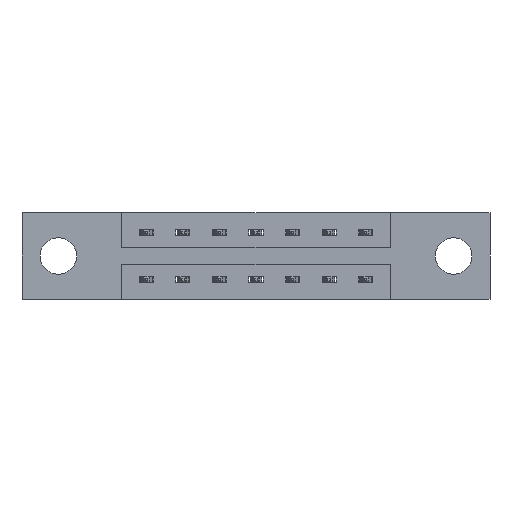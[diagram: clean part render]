
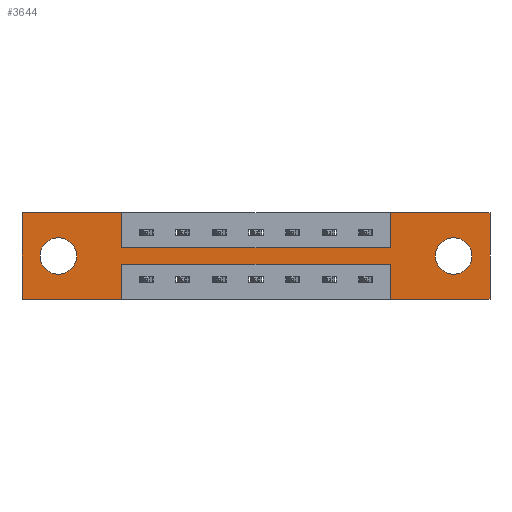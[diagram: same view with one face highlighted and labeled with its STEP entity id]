
A CAD part, front view. The second image highlights one B-rep face of the part: STEP entity #3644.
In plain terms, the highlighted planar face has unit normal (0, -1, 0).
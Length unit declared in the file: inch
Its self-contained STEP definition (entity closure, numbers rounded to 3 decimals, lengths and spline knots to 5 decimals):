
#55 = EDGE_CURVE ( 'NONE', #8489, #938, #3710, .T. ) ;
#57 = CIRCLE ( 'NONE', #2576, 0.078 ) ;
#244 = EDGE_CURVE ( 'NONE', #3128, #1356, #6852, .T. ) ;
#360 = DIRECTION ( 'NONE',  ( 0., 1., 0. ) ) ;
#415 = DIRECTION ( 'NONE',  ( 1., 0., 0. ) ) ;
#687 = CARTESIAN_POINT ( 'NONE',  ( 0.155, 0., -0.185 ) ) ;
#725 = ORIENTED_EDGE ( 'NONE', *, *, #8463, .F. ) ;
#742 = ORIENTED_EDGE ( 'NONE', *, *, #244, .F. ) ;
#936 = LINE ( 'NONE', #1928, #2148 ) ;
#938 = VERTEX_POINT ( 'NONE', #7588 ) ;
#1130 = VERTEX_POINT ( 'NONE', #7873 ) ;
#1139 = ORIENTED_EDGE ( 'NONE', *, *, #9358, .F. ) ;
#1258 = DIRECTION ( 'NONE',  ( 0., 0., -1. ) ) ;
#1273 = VERTEX_POINT ( 'NONE', #8137 ) ;
#1356 = VERTEX_POINT ( 'NONE', #8994 ) ;
#1363 = EDGE_CURVE ( 'NONE', #7851, #3679, #5012, .T. ) ;
#1532 = LINE ( 'NONE', #3522, #5230 ) ;
#1639 = DIRECTION ( 'NONE',  ( 0., 0., 1. ) ) ;
#1818 = EDGE_CURVE ( 'NONE', #1130, #3128, #1532, .T. ) ;
#1835 = CARTESIAN_POINT ( 'NONE',  ( 0.425, 0., -0.15 ) ) ;
#1843 = LINE ( 'NONE', #5251, #6759 ) ;
#1888 = CIRCLE ( 'NONE', #5124, 0.078 ) ;
#1928 = CARTESIAN_POINT ( 'NONE',  ( 1.573, 0., 0. ) ) ;
#2063 = LINE ( 'NONE', #8984, #8922 ) ;
#2148 = VECTOR ( 'NONE', #2625, 39.37008 ) ;
#2162 = CARTESIAN_POINT ( 'NONE',  ( 0., 0., -0.37 ) ) ;
#2202 = AXIS2_PLACEMENT_3D ( 'NONE', #687, #4536, #9292 ) ;
#2242 = DIRECTION ( 'NONE',  ( 0., 0., -1. ) ) ;
#2257 = FACE_BOUND ( 'NONE', #9758, .T. ) ;
#2281 = VERTEX_POINT ( 'NONE', #3507 ) ;
#2293 = VECTOR ( 'NONE', #8627, 39.37008 ) ;
#2341 = LINE ( 'NONE', #7814, #8841 ) ;
#2391 = VECTOR ( 'NONE', #5504, 39.37008 ) ;
#2440 = CARTESIAN_POINT ( 'NONE',  ( 1.573, 0., -0.37 ) ) ;
#2482 = VECTOR ( 'NONE', #4920, 39.37008 ) ;
#2576 = AXIS2_PLACEMENT_3D ( 'NONE', #2961, #6100, #4582 ) ;
#2597 = CARTESIAN_POINT ( 'NONE',  ( 0., 0., -0.37 ) ) ;
#2625 = DIRECTION ( 'NONE',  ( 0., 0., 1. ) ) ;
#2782 = VECTOR ( 'NONE', #5097, 39.37008 ) ;
#2894 = VERTEX_POINT ( 'NONE', #5723 ) ;
#2911 = EDGE_LOOP ( 'NONE', ( #9784, #5917 ) ) ;
#2961 = CARTESIAN_POINT ( 'NONE',  ( 0.155, 0., -0.185 ) ) ;
#2973 = ORIENTED_EDGE ( 'NONE', *, *, #6583, .F. ) ;
#3128 = VERTEX_POINT ( 'NONE', #8441 ) ;
#3323 = VECTOR ( 'NONE', #7646, 39.37008 ) ;
#3328 = AXIS2_PLACEMENT_3D ( 'NONE', #8236, #6020, #5959 ) ;
#3358 = VECTOR ( 'NONE', #8349, 39.37008 ) ;
#3507 = CARTESIAN_POINT ( 'NONE',  ( 1.573, 0., -0.15 ) ) ;
#3522 = CARTESIAN_POINT ( 'NONE',  ( 1.998, 0., 0. ) ) ;
#3532 = EDGE_CURVE ( 'NONE', #7318, #4775, #57, .T. ) ;
#3644 = ADVANCED_FACE ( 'NONE', ( #9954, #2257, #4858 ), #6828, .T. ) ;
#3679 = VERTEX_POINT ( 'NONE', #5228 ) ;
#3710 = LINE ( 'NONE', #8182, #2782 ) ;
#3792 = LINE ( 'NONE', #4571, #3323 ) ;
#4069 = ORIENTED_EDGE ( 'NONE', *, *, #9150, .F. ) ;
#4127 = CARTESIAN_POINT ( 'NONE',  ( 0., 0., 0. ) ) ;
#4367 = EDGE_CURVE ( 'NONE', #3679, #7851, #1888, .T. ) ;
#4536 = DIRECTION ( 'NONE',  ( 0., 1., 0. ) ) ;
#4571 = CARTESIAN_POINT ( 'NONE',  ( 0., 0., -0.37 ) ) ;
#4582 = DIRECTION ( 'NONE',  ( 0., 0., 1. ) ) ;
#4628 = EDGE_CURVE ( 'NONE', #4775, #7318, #9238, .T. ) ;
#4639 = ORIENTED_EDGE ( 'NONE', *, *, #1818, .F. ) ;
#4667 = CARTESIAN_POINT ( 'NONE',  ( 0., 0., 0. ) ) ;
#4775 = VERTEX_POINT ( 'NONE', #7078 ) ;
#4822 = CARTESIAN_POINT ( 'NONE',  ( 1.843, 0., -0.185 ) ) ;
#4858 = FACE_OUTER_BOUND ( 'NONE', #6739, .T. ) ;
#4920 = DIRECTION ( 'NONE',  ( 0., 0., 1. ) ) ;
#5012 = CIRCLE ( 'NONE', #3328, 0.078 ) ;
#5097 = DIRECTION ( 'NONE',  ( 1., 0., 0. ) ) ;
#5124 = AXIS2_PLACEMENT_3D ( 'NONE', #4822, #360, #7941 ) ;
#5191 = VERTEX_POINT ( 'NONE', #9258 ) ;
#5228 = CARTESIAN_POINT ( 'NONE',  ( 1.843, 0., -0.107 ) ) ;
#5230 = VECTOR ( 'NONE', #1258, 39.37008 ) ;
#5251 = CARTESIAN_POINT ( 'NONE',  ( 0., 0., 0. ) ) ;
#5385 = ORIENTED_EDGE ( 'NONE', *, *, #55, .F. ) ;
#5395 = EDGE_CURVE ( 'NONE', #6432, #8489, #7751, .T. ) ;
#5457 = ORIENTED_EDGE ( 'NONE', *, *, #4628, .T. ) ;
#5504 = DIRECTION ( 'NONE',  ( 0., 0., -1. ) ) ;
#5588 = CARTESIAN_POINT ( 'NONE',  ( 1.843, 0., -0.263 ) ) ;
#5723 = CARTESIAN_POINT ( 'NONE',  ( 0.425, 0., -0.22 ) ) ;
#5917 = ORIENTED_EDGE ( 'NONE', *, *, #1363, .T. ) ;
#5959 = DIRECTION ( 'NONE',  ( 0., 0., -1. ) ) ;
#6020 = DIRECTION ( 'NONE',  ( 0., 1., 0. ) ) ;
#6024 = ORIENTED_EDGE ( 'NONE', *, *, #9821, .F. ) ;
#6059 = EDGE_CURVE ( 'NONE', #938, #8451, #2341, .T. ) ;
#6100 = DIRECTION ( 'NONE',  ( 0., 1., 0. ) ) ;
#6432 = VERTEX_POINT ( 'NONE', #2597 ) ;
#6583 = EDGE_CURVE ( 'NONE', #9406, #1130, #1843, .T. ) ;
#6615 = LINE ( 'NONE', #7100, #2293 ) ;
#6739 = EDGE_LOOP ( 'NONE', ( #9679, #725, #6024, #742, #4639, #2973, #4069, #7630, #7072, #5385, #9112, #1139 ) ) ;
#6759 = VECTOR ( 'NONE', #8379, 39.37008 ) ;
#6828 = PLANE ( 'NONE',  #8109 ) ;
#6851 = CARTESIAN_POINT ( 'NONE',  ( 1.573, 0., 0. ) ) ;
#6852 = LINE ( 'NONE', #2162, #3358 ) ;
#6912 = VECTOR ( 'NONE', #1639, 39.37008 ) ;
#7030 = CARTESIAN_POINT ( 'NONE',  ( 0.425, 0., -0.37 ) ) ;
#7072 = ORIENTED_EDGE ( 'NONE', *, *, #6059, .F. ) ;
#7078 = CARTESIAN_POINT ( 'NONE',  ( 0.155, 0., -0.107 ) ) ;
#7100 = CARTESIAN_POINT ( 'NONE',  ( 0.425, 0., -0.22 ) ) ;
#7318 = VERTEX_POINT ( 'NONE', #7822 ) ;
#7373 = EDGE_CURVE ( 'NONE', #8451, #2281, #2063, .T. ) ;
#7552 = CARTESIAN_POINT ( 'NONE',  ( 0., 0., -0.37 ) ) ;
#7588 = CARTESIAN_POINT ( 'NONE',  ( 0.425, 0., 0. ) ) ;
#7630 = ORIENTED_EDGE ( 'NONE', *, *, #7373, .F. ) ;
#7646 = DIRECTION ( 'NONE',  ( -1., 0., 0. ) ) ;
#7656 = DIRECTION ( 'NONE',  ( 0., -1., 0. ) ) ;
#7751 = LINE ( 'NONE', #4667, #6912 ) ;
#7814 = CARTESIAN_POINT ( 'NONE',  ( 0.425, 0., 0. ) ) ;
#7822 = CARTESIAN_POINT ( 'NONE',  ( 0.155, 0., -0.263 ) ) ;
#7851 = VERTEX_POINT ( 'NONE', #5588 ) ;
#7873 = CARTESIAN_POINT ( 'NONE',  ( 1.998, 0., 0. ) ) ;
#7941 = DIRECTION ( 'NONE',  ( 0., 0., -1. ) ) ;
#8109 = AXIS2_PLACEMENT_3D ( 'NONE', #7552, #7656, #2242 ) ;
#8137 = CARTESIAN_POINT ( 'NONE',  ( 0.425, 0., -0.37 ) ) ;
#8182 = CARTESIAN_POINT ( 'NONE',  ( 0., 0., 0. ) ) ;
#8236 = CARTESIAN_POINT ( 'NONE',  ( 1.843, 0., -0.185 ) ) ;
#8349 = DIRECTION ( 'NONE',  ( -1., 0., 0. ) ) ;
#8379 = DIRECTION ( 'NONE',  ( 1., 0., 0. ) ) ;
#8409 = ORIENTED_EDGE ( 'NONE', *, *, #3532, .T. ) ;
#8441 = CARTESIAN_POINT ( 'NONE',  ( 1.998, 0., -0.37 ) ) ;
#8451 = VERTEX_POINT ( 'NONE', #1835 ) ;
#8463 = EDGE_CURVE ( 'NONE', #5191, #2894, #6615, .T. ) ;
#8489 = VERTEX_POINT ( 'NONE', #4127 ) ;
#8627 = DIRECTION ( 'NONE',  ( -1., 0., 0. ) ) ;
#8638 = DIRECTION ( 'NONE',  ( 0., 0., -1. ) ) ;
#8841 = VECTOR ( 'NONE', #8638, 39.37008 ) ;
#8922 = VECTOR ( 'NONE', #415, 39.37008 ) ;
#8984 = CARTESIAN_POINT ( 'NONE',  ( 0.425, 0., -0.15 ) ) ;
#8994 = CARTESIAN_POINT ( 'NONE',  ( 1.573, 0., -0.37 ) ) ;
#9018 = LINE ( 'NONE', #7030, #2391 ) ;
#9112 = ORIENTED_EDGE ( 'NONE', *, *, #5395, .F. ) ;
#9125 = EDGE_CURVE ( 'NONE', #2894, #1273, #9018, .T. ) ;
#9150 = EDGE_CURVE ( 'NONE', #2281, #9406, #936, .T. ) ;
#9238 = CIRCLE ( 'NONE', #2202, 0.078 ) ;
#9258 = CARTESIAN_POINT ( 'NONE',  ( 1.573, 0., -0.22 ) ) ;
#9292 = DIRECTION ( 'NONE',  ( 0., 0., 1. ) ) ;
#9358 = EDGE_CURVE ( 'NONE', #1273, #6432, #3792, .T. ) ;
#9406 = VERTEX_POINT ( 'NONE', #6851 ) ;
#9679 = ORIENTED_EDGE ( 'NONE', *, *, #9125, .F. ) ;
#9703 = LINE ( 'NONE', #2440, #2482 ) ;
#9758 = EDGE_LOOP ( 'NONE', ( #5457, #8409 ) ) ;
#9784 = ORIENTED_EDGE ( 'NONE', *, *, #4367, .T. ) ;
#9821 = EDGE_CURVE ( 'NONE', #1356, #5191, #9703, .T. ) ;
#9954 = FACE_BOUND ( 'NONE', #2911, .T. ) ;
